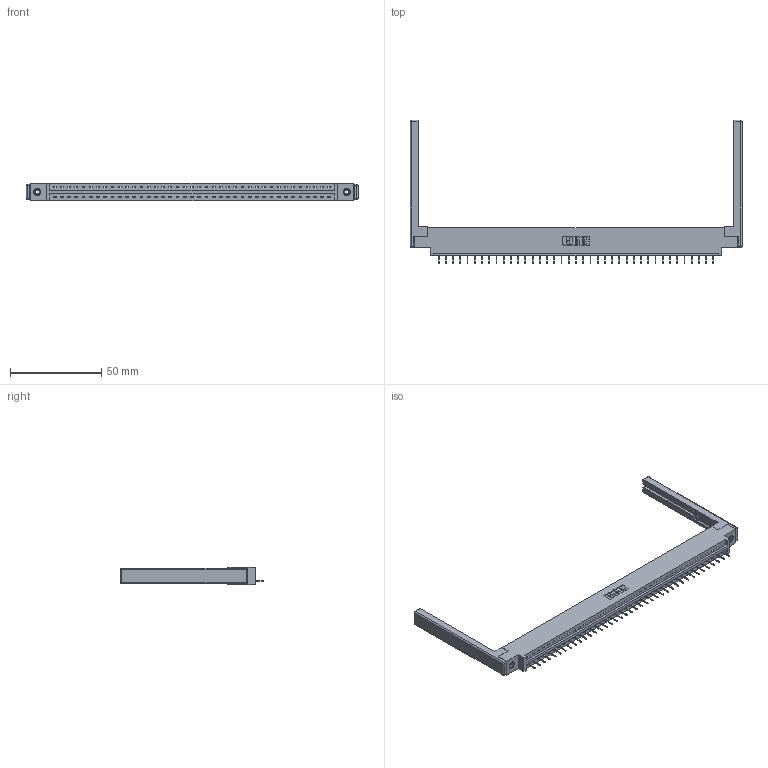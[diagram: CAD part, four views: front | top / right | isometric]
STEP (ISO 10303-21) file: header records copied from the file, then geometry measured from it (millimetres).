
FILE_DESCRIPTION (( 'STEP AP203' ), '1' );
FILE_NAME ('387-039-524-668.STEP', '2019-10-04T17:23:31', ( '' ), ( '' ), 'SwSTEP 2.0', 'SolidWorks 2016', '' );
FILE_SCHEMA (( 'CONFIG_CONTROL_DESIGN' ));
Length unit declared in the file: inch
Products named in the file (5): 345-250-001_345-250-001-102; 345-292-001_345-293-124; 337 Part_0.170 Offset - 0.156 Dia-TI; 387-039-524-668; 307-220-068
Assembly tree (44 placements, depth 2):
  387-039-524-668
    337 Part_0.170 Offset - 0.156 Dia-TI
    345-292-001_345-293-124  x39
    345-250-001_345-250-001-102  x2
    307-220-068  x2
Bounding box: 181.97 x 78.75 x 9.4 mm (x, y, z)
Volume: 22994.4 mm3; surface area: 22854.3 mm2
Topology: 44 solids, 44 shells, 2846 faces, 8201 edges, 5290 vertices
Faces by surface type: plane 2190, cylinder 632, cone 12, sphere 8, torus 4
Entity records: 32344 total; most frequent: CARTESIAN_POINT 5588, ORIENTED_EDGE 5552, DIRECTION 4784, EDGE_CURVE 2776, VECTOR 2602, LINE 2602, VERTEX_POINT 1838, AXIS2_PLACEMENT_3D 1091
